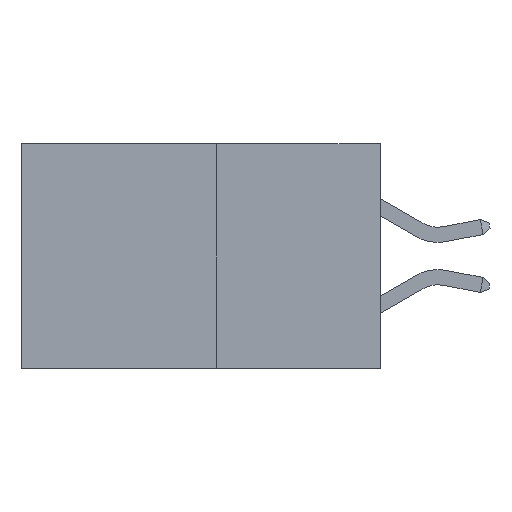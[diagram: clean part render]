
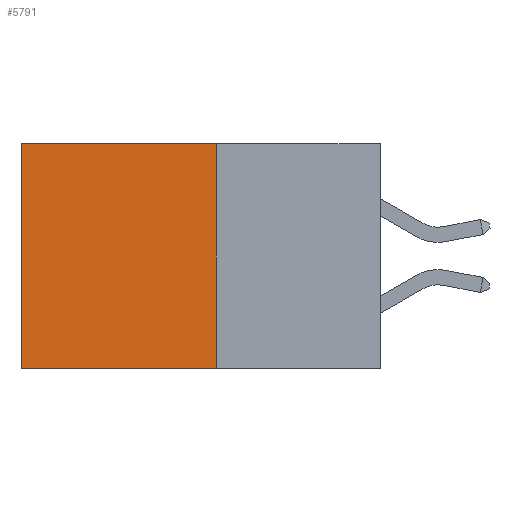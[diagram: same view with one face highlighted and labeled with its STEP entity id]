
A CAD part, left-side view. The second image highlights one B-rep face of the part: STEP entity #5791.
In plain terms, the highlighted planar face has unit normal (-1, 0, 0).
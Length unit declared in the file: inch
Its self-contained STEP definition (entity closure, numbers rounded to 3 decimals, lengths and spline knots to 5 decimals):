
#179 = DIRECTION ( 'NONE',  ( 0., 0., -1. ) ) ;
#198 = EDGE_CURVE ( 'NONE', #9905, #2612, #5852, .T. ) ;
#395 = CARTESIAN_POINT ( 'NONE',  ( 0.277, 0.27, -0.37 ) ) ;
#410 = CARTESIAN_POINT ( 'NONE',  ( 0.277, 0.59, -0.37 ) ) ;
#774 = EDGE_CURVE ( 'NONE', #2612, #6709, #7362, .T. ) ;
#1020 = VECTOR ( 'NONE', #2796, 39.37008 ) ;
#1638 = ORIENTED_EDGE ( 'NONE', *, *, #2895, .F. ) ;
#1988 = LINE ( 'NONE', #6824, #10584 ) ;
#2333 = CARTESIAN_POINT ( 'NONE',  ( 0.277, 0.59, -0.37 ) ) ;
#2444 = CARTESIAN_POINT ( 'NONE',  ( 0.277, 0.27, 0. ) ) ;
#2612 = VERTEX_POINT ( 'NONE', #7077 ) ;
#2796 = DIRECTION ( 'NONE',  ( 0., 1., 0. ) ) ;
#2895 = EDGE_CURVE ( 'NONE', #6145, #6709, #1988, .T. ) ;
#3008 = VECTOR ( 'NONE', #179, 39.37008 ) ;
#3181 = CARTESIAN_POINT ( 'NONE',  ( 0.277, 0.27, -0.37 ) ) ;
#3543 = EDGE_CURVE ( 'NONE', #9905, #6145, #9912, .T. ) ;
#4059 = DIRECTION ( 'NONE',  ( 1., 0., 0. ) ) ;
#5639 = DIRECTION ( 'NONE',  ( 0., 0., -1. ) ) ;
#5791 = ADVANCED_FACE ( 'NONE', ( #8549 ), #8257, .F. ) ;
#5852 = LINE ( 'NONE', #2444, #1020 ) ;
#6145 = VERTEX_POINT ( 'NONE', #9446 ) ;
#6468 = EDGE_LOOP ( 'NONE', ( #10085, #1638, #10321, #10090 ) ) ;
#6709 = VERTEX_POINT ( 'NONE', #410 ) ;
#6812 = DIRECTION ( 'NONE',  ( 0., 1., 0. ) ) ;
#6824 = CARTESIAN_POINT ( 'NONE',  ( 0.277, 0.27, -0.37 ) ) ;
#7077 = CARTESIAN_POINT ( 'NONE',  ( 0.277, 0.59, 0. ) ) ;
#7362 = LINE ( 'NONE', #2333, #3008 ) ;
#8257 = PLANE ( 'NONE',  #8551 ) ;
#8278 = VECTOR ( 'NONE', #5639, 39.37008 ) ;
#8549 = FACE_OUTER_BOUND ( 'NONE', #6468, .T. ) ;
#8551 = AXIS2_PLACEMENT_3D ( 'NONE', #3181, #4059, #9674 ) ;
#9446 = CARTESIAN_POINT ( 'NONE',  ( 0.277, 0.27, -0.37 ) ) ;
#9674 = DIRECTION ( 'NONE',  ( 0., 0., -1. ) ) ;
#9905 = VERTEX_POINT ( 'NONE', #10245 ) ;
#9912 = LINE ( 'NONE', #395, #8278 ) ;
#10085 = ORIENTED_EDGE ( 'NONE', *, *, #774, .T. ) ;
#10090 = ORIENTED_EDGE ( 'NONE', *, *, #198, .T. ) ;
#10245 = CARTESIAN_POINT ( 'NONE',  ( 0.277, 0.27, 0. ) ) ;
#10321 = ORIENTED_EDGE ( 'NONE', *, *, #3543, .F. ) ;
#10584 = VECTOR ( 'NONE', #6812, 39.37008 ) ;
